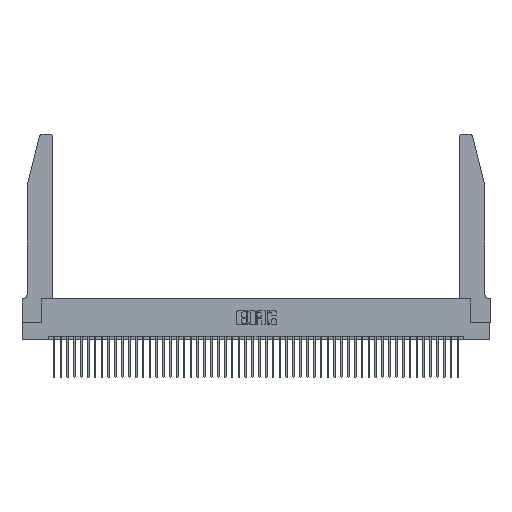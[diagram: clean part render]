
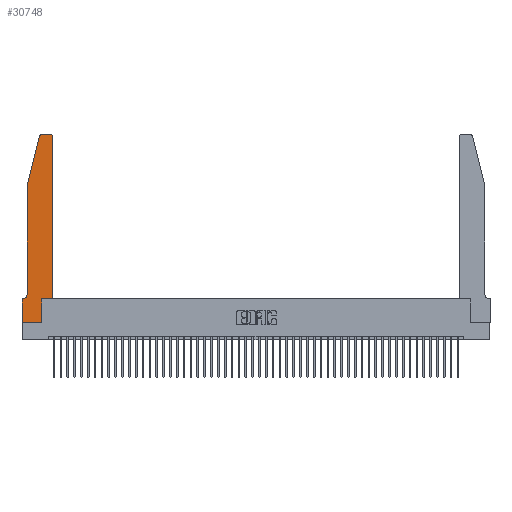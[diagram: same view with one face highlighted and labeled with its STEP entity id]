
A CAD part, top view. The second image highlights one B-rep face of the part: STEP entity #30748.
In plain terms, the highlighted planar face has unit normal (0, 0, 1).
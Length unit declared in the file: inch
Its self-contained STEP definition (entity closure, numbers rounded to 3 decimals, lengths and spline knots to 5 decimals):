
#898 = ORIENTED_EDGE ( 'NONE', *, *, #25875, .T. ) ;
#1406 = CARTESIAN_POINT ( 'NONE',  ( 0.284, 2.72, 0.37 ) ) ;
#1425 = VERTEX_POINT ( 'NONE', #29236 ) ;
#1581 = CARTESIAN_POINT ( 'NONE',  ( 0.284, 2.75, 0.37 ) ) ;
#1959 = EDGE_CURVE ( 'NONE', #40188, #37286, #30349, .T. ) ;
#2942 = LINE ( 'NONE', #8008, #12010 ) ;
#3203 = EDGE_LOOP ( 'NONE', ( #898, #29534, #6228, #34758, #4116, #8335, #31036, #31283, #13003, #13142, #32243, #9835 ) ) ;
#4116 = ORIENTED_EDGE ( 'NONE', *, *, #36217, .T. ) ;
#4332 = AXIS2_PLACEMENT_3D ( 'NONE', #7717, #34526, #11587 ) ;
#4994 = CARTESIAN_POINT ( 'NONE',  ( 0.4505, 0.35, 0.37 ) ) ;
#5181 = DIRECTION ( 'NONE',  ( 0., -1., 0. ) ) ;
#5268 = DIRECTION ( 'NONE',  ( 1., 0., 0. ) ) ;
#5343 = CARTESIAN_POINT ( 'NONE',  ( 0.0755, 2., 0.37 ) ) ;
#5883 = LINE ( 'NONE', #34402, #25186 ) ;
#6228 = ORIENTED_EDGE ( 'NONE', *, *, #7306, .T. ) ;
#6352 = VERTEX_POINT ( 'NONE', #13111 ) ;
#7298 = DIRECTION ( 'NONE',  ( -0.239, -0.971, 0. ) ) ;
#7306 = EDGE_CURVE ( 'NONE', #1425, #40188, #20737, .T. ) ;
#7338 = CARTESIAN_POINT ( 'NONE',  ( 0.2605, 2.75, 0.37 ) ) ;
#7717 = CARTESIAN_POINT ( 'NONE',  ( 0.4205, 2.72, 0.37 ) ) ;
#8008 = CARTESIAN_POINT ( 'NONE',  ( 0.4505, 0.35, 0.37 ) ) ;
#8335 = ORIENTED_EDGE ( 'NONE', *, *, #10366, .T. ) ;
#8604 = CARTESIAN_POINT ( 'NONE',  ( 0.2865, 0.35, 0.37 ) ) ;
#8984 = LINE ( 'NONE', #34004, #28258 ) ;
#9835 = ORIENTED_EDGE ( 'NONE', *, *, #23302, .T. ) ;
#9958 = VERTEX_POINT ( 'NONE', #1581 ) ;
#10011 = VECTOR ( 'NONE', #34843, 39.37008 ) ;
#10366 = EDGE_CURVE ( 'NONE', #20617, #37380, #5883, .T. ) ;
#10406 = VECTOR ( 'NONE', #7298, 39.37008 ) ;
#10880 = CARTESIAN_POINT ( 'NONE',  ( 0.4205, 2.75, 0.37 ) ) ;
#11145 = EDGE_CURVE ( 'NONE', #27077, #17541, #44672, .T. ) ;
#11274 = AXIS2_PLACEMENT_3D ( 'NONE', #1406, #28298, #5268 ) ;
#11587 = DIRECTION ( 'NONE',  ( 1., 0., 0. ) ) ;
#11915 = DIRECTION ( 'NONE',  ( 1., 0., 0. ) ) ;
#12010 = VECTOR ( 'NONE', #11915, 39.37008 ) ;
#12358 = FACE_OUTER_BOUND ( 'NONE', #3203, .T. ) ;
#13003 = ORIENTED_EDGE ( 'NONE', *, *, #11145, .T. ) ;
#13111 = CARTESIAN_POINT ( 'NONE',  ( 0.4505, 2.72, 0.37 ) ) ;
#13142 = ORIENTED_EDGE ( 'NONE', *, *, #41305, .T. ) ;
#15477 = CARTESIAN_POINT ( 'NONE',  ( 0.0055, 0.42, 0.37 ) ) ;
#15642 = AXIS2_PLACEMENT_3D ( 'NONE', #15477, #42179, #19390 ) ;
#15700 = CIRCLE ( 'NONE', #15642, 0.07 ) ;
#15920 = VECTOR ( 'NONE', #30327, 39.37008 ) ;
#16628 = EDGE_CURVE ( 'NONE', #37380, #23067, #27102, .T. ) ;
#16675 = CARTESIAN_POINT ( 'NONE',  ( 0.0055, 0.35, 0.37 ) ) ;
#17228 = CARTESIAN_POINT ( 'NONE',  ( 0., 0., 0.37 ) ) ;
#17541 = VERTEX_POINT ( 'NONE', #8604 ) ;
#17618 = EDGE_CURVE ( 'NONE', #9958, #1425, #23451, .T. ) ;
#18100 = VECTOR ( 'NONE', #32876, 39.37008 ) ;
#18706 = DIRECTION ( 'NONE',  ( 1., 0., 0. ) ) ;
#19025 = VECTOR ( 'NONE', #5181, 39.37008 ) ;
#19390 = DIRECTION ( 'NONE',  ( -1., 0., 0. ) ) ;
#19730 = CARTESIAN_POINT ( 'NONE',  ( 0., 0., 0.37 ) ) ;
#20617 = VERTEX_POINT ( 'NONE', #16675 ) ;
#20737 = LINE ( 'NONE', #37774, #10406 ) ;
#22746 = DIRECTION ( 'NONE',  ( 0., 1., 0. ) ) ;
#23067 = VERTEX_POINT ( 'NONE', #17228 ) ;
#23302 = EDGE_CURVE ( 'NONE', #6352, #29604, #43621, .T. ) ;
#23451 = CIRCLE ( 'NONE', #11274, 0.03 ) ;
#24950 = LINE ( 'NONE', #7338, #15920 ) ;
#25186 = VECTOR ( 'NONE', #38248, 39.37008 ) ;
#25875 = EDGE_CURVE ( 'NONE', #29604, #9958, #24950, .T. ) ;
#26314 = CARTESIAN_POINT ( 'NONE',  ( 0.0755, 0.42, 0.37 ) ) ;
#27077 = VERTEX_POINT ( 'NONE', #33879 ) ;
#27102 = LINE ( 'NONE', #36678, #18100 ) ;
#28258 = VECTOR ( 'NONE', #22746, 39.37008 ) ;
#28298 = DIRECTION ( 'NONE',  ( 0., 0., 1. ) ) ;
#29236 = CARTESIAN_POINT ( 'NONE',  ( 0.25487, 2.72718, 0.37 ) ) ;
#29534 = ORIENTED_EDGE ( 'NONE', *, *, #17618, .T. ) ;
#29604 = VERTEX_POINT ( 'NONE', #10880 ) ;
#30327 = DIRECTION ( 'NONE',  ( -1., 0., 0. ) ) ;
#30349 = LINE ( 'NONE', #5343, #19025 ) ;
#30748 = ADVANCED_FACE ( 'NONE', ( #12358 ), #45121, .T. ) ;
#31036 = ORIENTED_EDGE ( 'NONE', *, *, #16628, .T. ) ;
#31044 = VERTEX_POINT ( 'NONE', #4994 ) ;
#31283 = ORIENTED_EDGE ( 'NONE', *, *, #42914, .T. ) ;
#31353 = DIRECTION ( 'NONE',  ( 0., 1., 0. ) ) ;
#31654 = LINE ( 'NONE', #19730, #10011 ) ;
#32243 = ORIENTED_EDGE ( 'NONE', *, *, #41162, .T. ) ;
#32876 = DIRECTION ( 'NONE',  ( 0., -1., 0. ) ) ;
#33853 = CARTESIAN_POINT ( 'NONE',  ( 0., 0.35, 0.37 ) ) ;
#33879 = CARTESIAN_POINT ( 'NONE',  ( 0.2865, 0., 0.37 ) ) ;
#34004 = CARTESIAN_POINT ( 'NONE',  ( 0.4505, 0.35, 0.37 ) ) ;
#34402 = CARTESIAN_POINT ( 'NONE',  ( 0.0755, 0.35, 0.37 ) ) ;
#34526 = DIRECTION ( 'NONE',  ( 0., 0., 1. ) ) ;
#34758 = ORIENTED_EDGE ( 'NONE', *, *, #1959, .T. ) ;
#34843 = DIRECTION ( 'NONE',  ( 1., 0., 0. ) ) ;
#36217 = EDGE_CURVE ( 'NONE', #37286, #20617, #15700, .T. ) ;
#36678 = CARTESIAN_POINT ( 'NONE',  ( 0., 0., 0.37 ) ) ;
#37286 = VERTEX_POINT ( 'NONE', #26314 ) ;
#37380 = VERTEX_POINT ( 'NONE', #42083 ) ;
#37774 = CARTESIAN_POINT ( 'NONE',  ( 0.0755, 2., 0.37 ) ) ;
#38248 = DIRECTION ( 'NONE',  ( -1., 0., 0. ) ) ;
#38847 = CARTESIAN_POINT ( 'NONE',  ( 0.2865, 0.35, 0.37 ) ) ;
#40188 = VERTEX_POINT ( 'NONE', #43739 ) ;
#41162 = EDGE_CURVE ( 'NONE', #31044, #6352, #8984, .T. ) ;
#41305 = EDGE_CURVE ( 'NONE', #17541, #31044, #2942, .T. ) ;
#41521 = DIRECTION ( 'NONE',  ( 0., 0., 1. ) ) ;
#42083 = CARTESIAN_POINT ( 'NONE',  ( 0., 0.35, 0.37 ) ) ;
#42179 = DIRECTION ( 'NONE',  ( 0., 0., -1. ) ) ;
#42914 = EDGE_CURVE ( 'NONE', #23067, #27077, #31654, .T. ) ;
#43521 = VECTOR ( 'NONE', #31353, 39.37008 ) ;
#43621 = CIRCLE ( 'NONE', #4332, 0.03 ) ;
#43739 = CARTESIAN_POINT ( 'NONE',  ( 0.0755, 2., 0.37 ) ) ;
#44672 = LINE ( 'NONE', #38847, #43521 ) ;
#45121 = PLANE ( 'NONE',  #48320 ) ;
#48320 = AXIS2_PLACEMENT_3D ( 'NONE', #33853, #41521, #18706 ) ;
